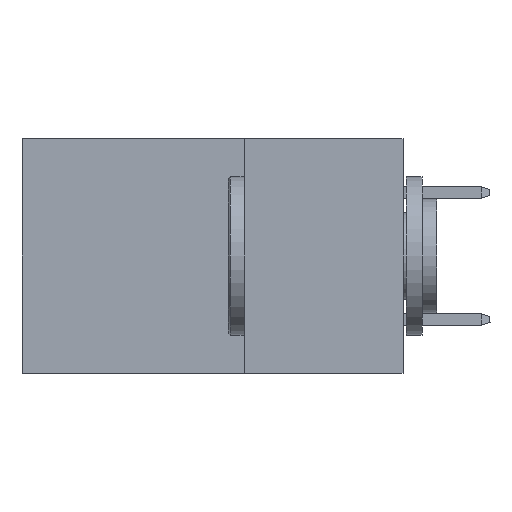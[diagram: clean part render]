
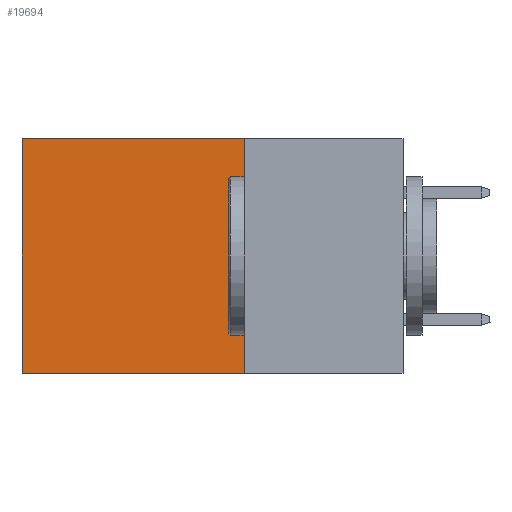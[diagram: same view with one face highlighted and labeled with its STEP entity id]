
A CAD part, left-side view. The second image highlights one B-rep face of the part: STEP entity #19694.
In plain terms, the highlighted planar face has unit normal (-1, 0, 0).
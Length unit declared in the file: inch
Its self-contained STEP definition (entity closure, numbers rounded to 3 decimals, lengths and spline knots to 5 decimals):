
#1423 = CARTESIAN_POINT ( 'NONE',  ( 0.2875, 0.25, 0. ) ) ;
#2141 = DIRECTION ( 'NONE',  ( 0., 1., 0. ) ) ;
#3056 = CARTESIAN_POINT ( 'NONE',  ( 0.2875, 0.25, 0. ) ) ;
#3111 = CARTESIAN_POINT ( 'NONE',  ( 0.2875, 0.25, 0. ) ) ;
#3275 = DIRECTION ( 'NONE',  ( 0., 1., 0. ) ) ;
#3586 = PLANE ( 'NONE',  #19341 ) ;
#4093 = ORIENTED_EDGE ( 'NONE', *, *, #13533, .T. ) ;
#4294 = ORIENTED_EDGE ( 'NONE', *, *, #25192, .T. ) ;
#4388 = EDGE_CURVE ( 'NONE', #19149, #8316, #20066, .T. ) ;
#4884 = DIRECTION ( 'NONE',  ( 0., 0., -1. ) ) ;
#5820 = CARTESIAN_POINT ( 'NONE',  ( 0.2875, 0.25, -0.37 ) ) ;
#7868 = VECTOR ( 'NONE', #4884, 39.37008 ) ;
#8314 = VECTOR ( 'NONE', #20569, 39.37008 ) ;
#8316 = VERTEX_POINT ( 'NONE', #21623 ) ;
#8393 = CARTESIAN_POINT ( 'NONE',  ( 0.2875, 0.6, 0. ) ) ;
#9076 = DIRECTION ( 'NONE',  ( 0., 0., -1. ) ) ;
#10951 = EDGE_LOOP ( 'NONE', ( #4093, #25556, #16812, #4294 ) ) ;
#11328 = CARTESIAN_POINT ( 'NONE',  ( 0.2875, 0.6, 0. ) ) ;
#13157 = EDGE_CURVE ( 'NONE', #23680, #19149, #22831, .T. ) ;
#13533 = EDGE_CURVE ( 'NONE', #21423, #8316, #14543, .T. ) ;
#13579 = LINE ( 'NONE', #1423, #15912 ) ;
#14313 = CARTESIAN_POINT ( 'NONE',  ( 0.2875, 0.25, -0.37 ) ) ;
#14543 = LINE ( 'NONE', #11328, #8314 ) ;
#15912 = VECTOR ( 'NONE', #3275, 39.37008 ) ;
#16812 = ORIENTED_EDGE ( 'NONE', *, *, #13157, .F. ) ;
#17303 = DIRECTION ( 'NONE',  ( 1., 0., 0. ) ) ;
#17435 = CARTESIAN_POINT ( 'NONE',  ( 0.2875, 0.25, 0. ) ) ;
#18683 = VECTOR ( 'NONE', #2141, 39.37008 ) ;
#19149 = VERTEX_POINT ( 'NONE', #14313 ) ;
#19341 = AXIS2_PLACEMENT_3D ( 'NONE', #17435, #17303, #9076 ) ;
#19694 = ADVANCED_FACE ( 'NONE', ( #25091 ), #3586, .F. ) ;
#20066 = LINE ( 'NONE', #5820, #18683 ) ;
#20569 = DIRECTION ( 'NONE',  ( 0., 0., -1. ) ) ;
#21423 = VERTEX_POINT ( 'NONE', #8393 ) ;
#21623 = CARTESIAN_POINT ( 'NONE',  ( 0.2875, 0.6, -0.37 ) ) ;
#22831 = LINE ( 'NONE', #3056, #7868 ) ;
#23680 = VERTEX_POINT ( 'NONE', #3111 ) ;
#25091 = FACE_OUTER_BOUND ( 'NONE', #10951, .T. ) ;
#25192 = EDGE_CURVE ( 'NONE', #23680, #21423, #13579, .T. ) ;
#25556 = ORIENTED_EDGE ( 'NONE', *, *, #4388, .F. ) ;
